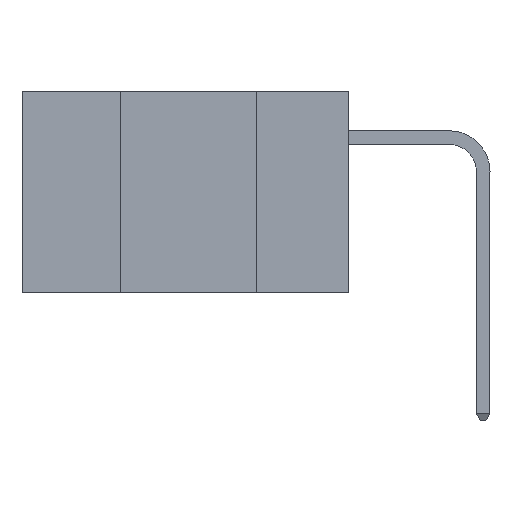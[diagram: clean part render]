
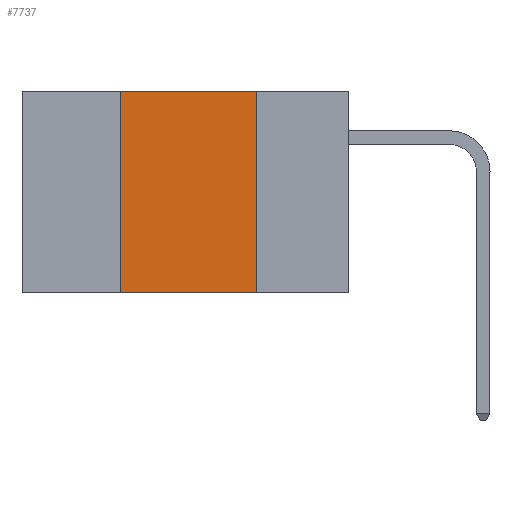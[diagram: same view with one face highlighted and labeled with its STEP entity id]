
A CAD part, left-side view. The second image highlights one B-rep face of the part: STEP entity #7737.
In plain terms, the highlighted planar face has unit normal (-1, 0, 0).
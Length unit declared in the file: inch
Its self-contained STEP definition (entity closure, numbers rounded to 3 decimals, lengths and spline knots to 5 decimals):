
#42 = VECTOR ( 'NONE', #20448, 39.37008 ) ;
#66 = ORIENTED_EDGE ( 'NONE', *, *, #32957, .F. ) ;
#570 = EDGE_CURVE ( 'NONE', #22286, #25329, #12719, .T. ) ;
#2188 = CARTESIAN_POINT ( 'NONE',  ( 0., 0.42, 0. ) ) ;
#2417 = CARTESIAN_POINT ( 'NONE',  ( 0., 0.17, 0. ) ) ;
#2705 = CARTESIAN_POINT ( 'NONE',  ( 0., 0.6, 0. ) ) ;
#4059 = CARTESIAN_POINT ( 'NONE',  ( 0., 0.6, -0.37 ) ) ;
#4899 = VERTEX_POINT ( 'NONE', #28198 ) ;
#7608 = CARTESIAN_POINT ( 'NONE',  ( 0., 0.42, 0. ) ) ;
#7737 = ADVANCED_FACE ( 'NONE', ( #13555 ), #25559, .F. ) ;
#8332 = LINE ( 'NONE', #2417, #13749 ) ;
#8758 = ORIENTED_EDGE ( 'NONE', *, *, #23441, .T. ) ;
#8883 = VERTEX_POINT ( 'NONE', #25172 ) ;
#9973 = EDGE_LOOP ( 'NONE', ( #9975, #18574, #66, #8758 ) ) ;
#9975 = ORIENTED_EDGE ( 'NONE', *, *, #23682, .F. ) ;
#11872 = VECTOR ( 'NONE', #16022, 39.37008 ) ;
#12719 = LINE ( 'NONE', #2705, #11872 ) ;
#12721 = DIRECTION ( 'NONE',  ( 0., 0., -1. ) ) ;
#13555 = FACE_OUTER_BOUND ( 'NONE', #9973, .T. ) ;
#13749 = VECTOR ( 'NONE', #30947, 39.37008 ) ;
#14145 = LINE ( 'NONE', #2188, #42 ) ;
#16022 = DIRECTION ( 'NONE',  ( 0., -1., 0. ) ) ;
#18574 = ORIENTED_EDGE ( 'NONE', *, *, #570, .F. ) ;
#19002 = CARTESIAN_POINT ( 'NONE',  ( 0., 0.17, 0. ) ) ;
#20398 = CARTESIAN_POINT ( 'NONE',  ( 0., 0.6, 0. ) ) ;
#20448 = DIRECTION ( 'NONE',  ( 0., 0., 1. ) ) ;
#22286 = VERTEX_POINT ( 'NONE', #7608 ) ;
#22383 = DIRECTION ( 'NONE',  ( 0., -1., 0. ) ) ;
#23430 = LINE ( 'NONE', #4059, #29445 ) ;
#23441 = EDGE_CURVE ( 'NONE', #8883, #4899, #23430, .T. ) ;
#23682 = EDGE_CURVE ( 'NONE', #25329, #4899, #8332, .T. ) ;
#25172 = CARTESIAN_POINT ( 'NONE',  ( 0., 0.42, -0.37 ) ) ;
#25329 = VERTEX_POINT ( 'NONE', #19002 ) ;
#25559 = PLANE ( 'NONE',  #33163 ) ;
#28120 = DIRECTION ( 'NONE',  ( 1., 0., 0. ) ) ;
#28198 = CARTESIAN_POINT ( 'NONE',  ( 0., 0.17, -0.37 ) ) ;
#29445 = VECTOR ( 'NONE', #22383, 39.37008 ) ;
#30947 = DIRECTION ( 'NONE',  ( 0., 0., -1. ) ) ;
#32957 = EDGE_CURVE ( 'NONE', #8883, #22286, #14145, .T. ) ;
#33163 = AXIS2_PLACEMENT_3D ( 'NONE', #20398, #28120, #12721 ) ;
